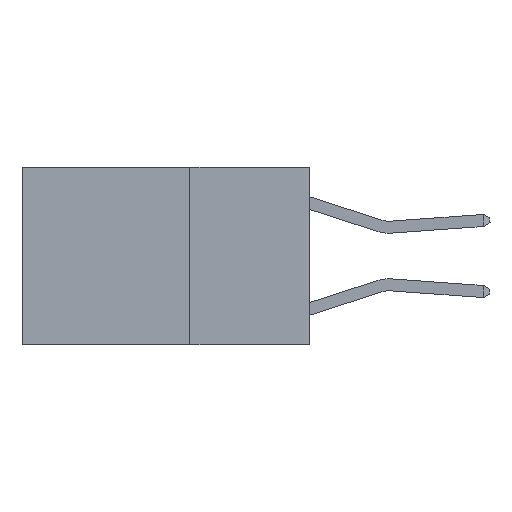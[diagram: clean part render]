
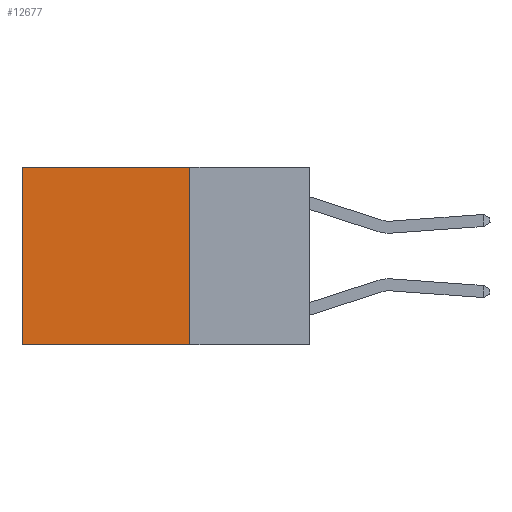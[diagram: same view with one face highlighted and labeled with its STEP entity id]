
A CAD part, left-side view. The second image highlights one B-rep face of the part: STEP entity #12677.
In plain terms, the highlighted planar face has unit normal (-1, 0, 0).
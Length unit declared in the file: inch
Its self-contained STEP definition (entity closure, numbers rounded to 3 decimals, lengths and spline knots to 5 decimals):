
#55 = EDGE_CURVE ( 'NONE', #4714, #4590, #13698, .T. ) ;
#816 = PLANE ( 'NONE',  #11443 ) ;
#1964 = EDGE_LOOP ( 'NONE', ( #11964, #3457, #3708, #4780 ) ) ;
#2094 = CARTESIAN_POINT ( 'NONE',  ( 0.2625, 0.25, -0.37 ) ) ;
#2311 = CARTESIAN_POINT ( 'NONE',  ( 0.2625, 0.6, 0. ) ) ;
#2334 = VECTOR ( 'NONE', #8998, 39.37008 ) ;
#3023 = LINE ( 'NONE', #7667, #11923 ) ;
#3110 = DIRECTION ( 'NONE',  ( 0., 0., -1. ) ) ;
#3457 = ORIENTED_EDGE ( 'NONE', *, *, #6968, .F. ) ;
#3508 = DIRECTION ( 'NONE',  ( 0., 0., -1. ) ) ;
#3708 = ORIENTED_EDGE ( 'NONE', *, *, #55, .F. ) ;
#4372 = DIRECTION ( 'NONE',  ( 0., 1., 0. ) ) ;
#4590 = VERTEX_POINT ( 'NONE', #11765 ) ;
#4714 = VERTEX_POINT ( 'NONE', #10888 ) ;
#4780 = ORIENTED_EDGE ( 'NONE', *, *, #6948, .T. ) ;
#5635 = VECTOR ( 'NONE', #4372, 39.37008 ) ;
#5645 = CARTESIAN_POINT ( 'NONE',  ( 0.2625, 0.6, 0. ) ) ;
#5653 = LINE ( 'NONE', #2311, #2334 ) ;
#6948 = EDGE_CURVE ( 'NONE', #4714, #9435, #3023, .T. ) ;
#6968 = EDGE_CURVE ( 'NONE', #4590, #12275, #11564, .T. ) ;
#7185 = CARTESIAN_POINT ( 'NONE',  ( 0.2625, 0.25, 0. ) ) ;
#7667 = CARTESIAN_POINT ( 'NONE',  ( 0.2625, 0.25, 0. ) ) ;
#8670 = CARTESIAN_POINT ( 'NONE',  ( 0.2625, 0.25, 0. ) ) ;
#8782 = DIRECTION ( 'NONE',  ( 0., 1., 0. ) ) ;
#8998 = DIRECTION ( 'NONE',  ( 0., 0., -1. ) ) ;
#9435 = VERTEX_POINT ( 'NONE', #5645 ) ;
#9801 = DIRECTION ( 'NONE',  ( 1., 0., 0. ) ) ;
#10135 = EDGE_CURVE ( 'NONE', #9435, #12275, #5653, .T. ) ;
#10201 = CARTESIAN_POINT ( 'NONE',  ( 0.2625, 0.6, -0.37 ) ) ;
#10888 = CARTESIAN_POINT ( 'NONE',  ( 0.2625, 0.25, 0. ) ) ;
#11092 = VECTOR ( 'NONE', #3508, 39.37008 ) ;
#11335 = FACE_OUTER_BOUND ( 'NONE', #1964, .T. ) ;
#11443 = AXIS2_PLACEMENT_3D ( 'NONE', #8670, #9801, #3110 ) ;
#11564 = LINE ( 'NONE', #2094, #5635 ) ;
#11765 = CARTESIAN_POINT ( 'NONE',  ( 0.2625, 0.25, -0.37 ) ) ;
#11923 = VECTOR ( 'NONE', #8782, 39.37008 ) ;
#11964 = ORIENTED_EDGE ( 'NONE', *, *, #10135, .T. ) ;
#12275 = VERTEX_POINT ( 'NONE', #10201 ) ;
#12677 = ADVANCED_FACE ( 'NONE', ( #11335 ), #816, .F. ) ;
#13698 = LINE ( 'NONE', #7185, #11092 ) ;
